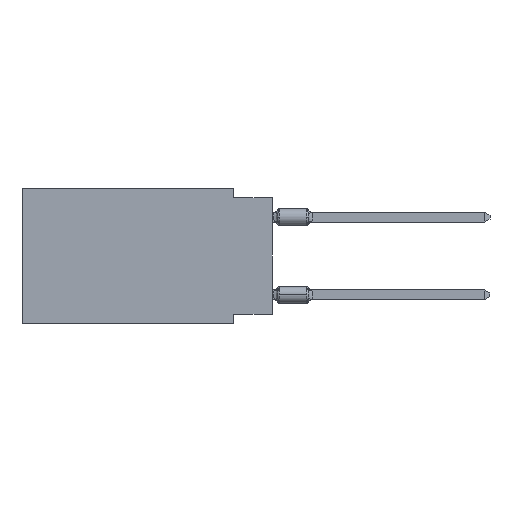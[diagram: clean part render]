
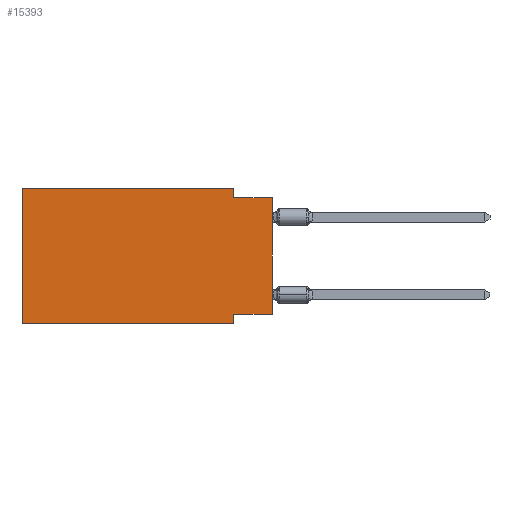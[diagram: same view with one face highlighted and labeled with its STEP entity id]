
A CAD part, left-side view. The second image highlights one B-rep face of the part: STEP entity #15393.
In plain terms, the highlighted planar face has unit normal (-1, 0, 0).
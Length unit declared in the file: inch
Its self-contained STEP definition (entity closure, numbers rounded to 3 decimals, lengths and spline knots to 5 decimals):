
#335 = CARTESIAN_POINT ( 'NONE',  ( 0., 0.645, 0. ) ) ;
#429 = DIRECTION ( 'NONE',  ( 0., -1., 0. ) ) ;
#1164 = DIRECTION ( 'NONE',  ( 0., -1., 0. ) ) ;
#1274 = VERTEX_POINT ( 'NONE', #18950 ) ;
#1664 = ORIENTED_EDGE ( 'NONE', *, *, #20436, .F. ) ;
#1726 = EDGE_CURVE ( 'NONE', #8211, #17821, #8997, .T. ) ;
#1745 = LINE ( 'NONE', #6429, #19245 ) ;
#1758 = ORIENTED_EDGE ( 'NONE', *, *, #8743, .T. ) ;
#1874 = LINE ( 'NONE', #3521, #15126 ) ;
#1951 = LINE ( 'NONE', #8589, #7513 ) ;
#2037 = EDGE_CURVE ( 'NONE', #1274, #2453, #3445, .T. ) ;
#2193 = ORIENTED_EDGE ( 'NONE', *, *, #1726, .F. ) ;
#2453 = VERTEX_POINT ( 'NONE', #335 ) ;
#3065 = DIRECTION ( 'NONE',  ( 0., 0., 1. ) ) ;
#3185 = EDGE_LOOP ( 'NONE', ( #18824, #19082, #2193, #8213, #14848, #1758, #1664, #10081 ) ) ;
#3275 = LINE ( 'NONE', #20140, #19017 ) ;
#3445 = LINE ( 'NONE', #16729, #18498 ) ;
#3483 = VERTEX_POINT ( 'NONE', #8584 ) ;
#3521 = CARTESIAN_POINT ( 'NONE',  ( 0., 0.1, -0.35 ) ) ;
#4543 = EDGE_CURVE ( 'NONE', #7119, #13173, #1745, .T. ) ;
#5606 = VECTOR ( 'NONE', #10518, 39.37008 ) ;
#5652 = DIRECTION ( 'NONE',  ( 1., 0., 0. ) ) ;
#6428 = DIRECTION ( 'NONE',  ( 0., -1., 0. ) ) ;
#6429 = CARTESIAN_POINT ( 'NONE',  ( 0., 0., 0. ) ) ;
#7119 = VERTEX_POINT ( 'NONE', #9603 ) ;
#7513 = VECTOR ( 'NONE', #429, 39.37008 ) ;
#7830 = EDGE_CURVE ( 'NONE', #17821, #13173, #11080, .T. ) ;
#8189 = CARTESIAN_POINT ( 'NONE',  ( 0., 0., -0.025 ) ) ;
#8211 = VERTEX_POINT ( 'NONE', #14308 ) ;
#8213 = ORIENTED_EDGE ( 'NONE', *, *, #8847, .F. ) ;
#8584 = CARTESIAN_POINT ( 'NONE',  ( 0., 0.1, -0.35 ) ) ;
#8589 = CARTESIAN_POINT ( 'NONE',  ( 0., 0.645, 0. ) ) ;
#8743 = EDGE_CURVE ( 'NONE', #1274, #3483, #3275, .T. ) ;
#8805 = CARTESIAN_POINT ( 'NONE',  ( 0., 0.1, -0.325 ) ) ;
#8847 = EDGE_CURVE ( 'NONE', #2453, #8211, #1951, .T. ) ;
#8997 = LINE ( 'NONE', #14009, #5606 ) ;
#9603 = CARTESIAN_POINT ( 'NONE',  ( 0., 0., -0.325 ) ) ;
#9750 = CARTESIAN_POINT ( 'NONE',  ( 0., 0.1, -0.025 ) ) ;
#10081 = ORIENTED_EDGE ( 'NONE', *, *, #11513, .F. ) ;
#10518 = DIRECTION ( 'NONE',  ( 0., 0., -1. ) ) ;
#10791 = VERTEX_POINT ( 'NONE', #8805 ) ;
#11080 = LINE ( 'NONE', #14559, #11336 ) ;
#11336 = VECTOR ( 'NONE', #1164, 39.37008 ) ;
#11513 = EDGE_CURVE ( 'NONE', #7119, #10791, #16435, .T. ) ;
#12424 = FACE_OUTER_BOUND ( 'NONE', #3185, .T. ) ;
#12632 = PLANE ( 'NONE',  #18981 ) ;
#13173 = VERTEX_POINT ( 'NONE', #8189 ) ;
#13735 = DIRECTION ( 'NONE',  ( 0., 0., -1. ) ) ;
#14009 = CARTESIAN_POINT ( 'NONE',  ( 0., 0.1, 0. ) ) ;
#14308 = CARTESIAN_POINT ( 'NONE',  ( 0., 0.1, 0. ) ) ;
#14559 = CARTESIAN_POINT ( 'NONE',  ( 0., 0., -0.025 ) ) ;
#14848 = ORIENTED_EDGE ( 'NONE', *, *, #2037, .F. ) ;
#15094 = DIRECTION ( 'NONE',  ( 0., 0., 1. ) ) ;
#15126 = VECTOR ( 'NONE', #13735, 39.37008 ) ;
#15393 = ADVANCED_FACE ( 'NONE', ( #12424 ), #12632, .F. ) ;
#15794 = DIRECTION ( 'NONE',  ( 0., 0., -1. ) ) ;
#16011 = CARTESIAN_POINT ( 'NONE',  ( 0., 0.645, 0. ) ) ;
#16435 = LINE ( 'NONE', #21142, #18126 ) ;
#16541 = DIRECTION ( 'NONE',  ( 0., 1., 0. ) ) ;
#16729 = CARTESIAN_POINT ( 'NONE',  ( 0., 0.645, 0. ) ) ;
#17821 = VERTEX_POINT ( 'NONE', #9750 ) ;
#18126 = VECTOR ( 'NONE', #16541, 39.37008 ) ;
#18498 = VECTOR ( 'NONE', #15094, 39.37008 ) ;
#18824 = ORIENTED_EDGE ( 'NONE', *, *, #4543, .T. ) ;
#18950 = CARTESIAN_POINT ( 'NONE',  ( 0., 0.645, -0.35 ) ) ;
#18981 = AXIS2_PLACEMENT_3D ( 'NONE', #16011, #5652, #15794 ) ;
#19017 = VECTOR ( 'NONE', #6428, 39.37008 ) ;
#19082 = ORIENTED_EDGE ( 'NONE', *, *, #7830, .F. ) ;
#19245 = VECTOR ( 'NONE', #3065, 39.37008 ) ;
#20140 = CARTESIAN_POINT ( 'NONE',  ( 0., 0.645, -0.35 ) ) ;
#20436 = EDGE_CURVE ( 'NONE', #10791, #3483, #1874, .T. ) ;
#21142 = CARTESIAN_POINT ( 'NONE',  ( 0., 0., -0.325 ) ) ;
